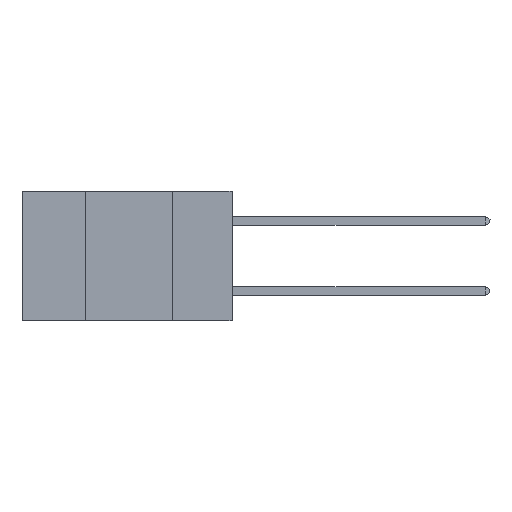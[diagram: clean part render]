
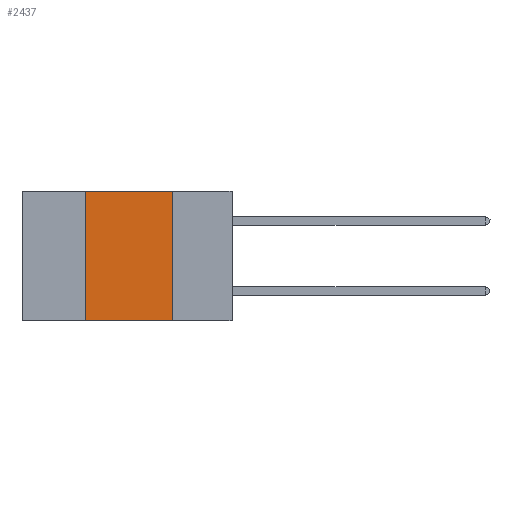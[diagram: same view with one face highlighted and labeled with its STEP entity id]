
A CAD part, left-side view. The second image highlights one B-rep face of the part: STEP entity #2437.
In plain terms, the highlighted planar face has unit normal (-1, 0, 0).
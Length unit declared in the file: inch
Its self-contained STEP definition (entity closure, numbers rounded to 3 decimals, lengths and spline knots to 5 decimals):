
#869 = PLANE ( 'NONE',  #8970 ) ;
#2437 = ADVANCED_FACE ( 'NONE', ( #35620 ), #869, .F. ) ;
#3408 = CARTESIAN_POINT ( 'NONE',  ( 0., 0.17, 0. ) ) ;
#4207 = VERTEX_POINT ( 'NONE', #16534 ) ;
#4420 = DIRECTION ( 'NONE',  ( 1., 0., 0. ) ) ;
#5138 = VECTOR ( 'NONE', #32113, 39.37008 ) ;
#7101 = EDGE_LOOP ( 'NONE', ( #16493, #40504, #42278, #21046 ) ) ;
#7404 = VERTEX_POINT ( 'NONE', #27531 ) ;
#7744 = CARTESIAN_POINT ( 'NONE',  ( 0., 0.6, 0. ) ) ;
#8970 = AXIS2_PLACEMENT_3D ( 'NONE', #7744, #4420, #28710 ) ;
#9797 = CARTESIAN_POINT ( 'NONE',  ( 0., 0.42, -0.37 ) ) ;
#10242 = VERTEX_POINT ( 'NONE', #9797 ) ;
#10516 = EDGE_CURVE ( 'NONE', #10242, #39474, #31238, .T. ) ;
#13121 = EDGE_CURVE ( 'NONE', #39474, #4207, #38425, .T. ) ;
#14902 = DIRECTION ( 'NONE',  ( 0., -1., 0. ) ) ;
#15189 = EDGE_CURVE ( 'NONE', #4207, #7404, #35589, .T. ) ;
#16493 = ORIENTED_EDGE ( 'NONE', *, *, #15189, .F. ) ;
#16534 = CARTESIAN_POINT ( 'NONE',  ( 0., 0.17, 0. ) ) ;
#18143 = CARTESIAN_POINT ( 'NONE',  ( 0., 0.42, 0. ) ) ;
#21046 = ORIENTED_EDGE ( 'NONE', *, *, #41332, .T. ) ;
#22135 = VECTOR ( 'NONE', #42083, 39.37008 ) ;
#27531 = CARTESIAN_POINT ( 'NONE',  ( 0., 0.17, -0.37 ) ) ;
#28701 = CARTESIAN_POINT ( 'NONE',  ( 0., 0.6, -0.37 ) ) ;
#28710 = DIRECTION ( 'NONE',  ( 0., 0., -1. ) ) ;
#29407 = VECTOR ( 'NONE', #14902, 39.37008 ) ;
#31238 = LINE ( 'NONE', #18143, #22135 ) ;
#32113 = DIRECTION ( 'NONE',  ( 0., -1., 0. ) ) ;
#32135 = CARTESIAN_POINT ( 'NONE',  ( 0., 0.6, 0. ) ) ;
#34508 = VECTOR ( 'NONE', #41338, 39.37008 ) ;
#35589 = LINE ( 'NONE', #3408, #34508 ) ;
#35620 = FACE_OUTER_BOUND ( 'NONE', #7101, .T. ) ;
#38425 = LINE ( 'NONE', #32135, #29407 ) ;
#39474 = VERTEX_POINT ( 'NONE', #41136 ) ;
#40504 = ORIENTED_EDGE ( 'NONE', *, *, #13121, .F. ) ;
#41136 = CARTESIAN_POINT ( 'NONE',  ( 0., 0.42, 0. ) ) ;
#41332 = EDGE_CURVE ( 'NONE', #10242, #7404, #41743, .T. ) ;
#41338 = DIRECTION ( 'NONE',  ( 0., 0., -1. ) ) ;
#41743 = LINE ( 'NONE', #28701, #5138 ) ;
#42083 = DIRECTION ( 'NONE',  ( 0., 0., 1. ) ) ;
#42278 = ORIENTED_EDGE ( 'NONE', *, *, #10516, .F. ) ;
